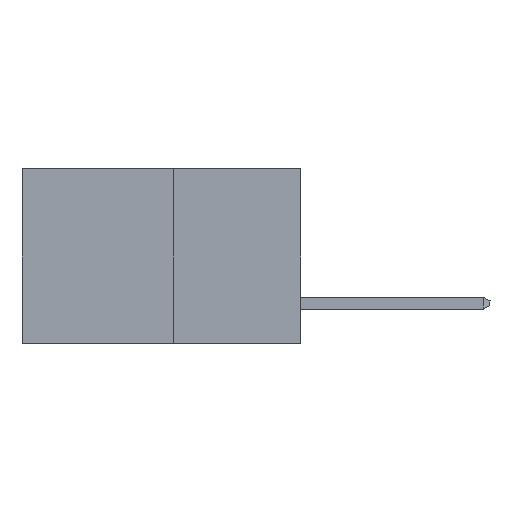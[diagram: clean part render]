
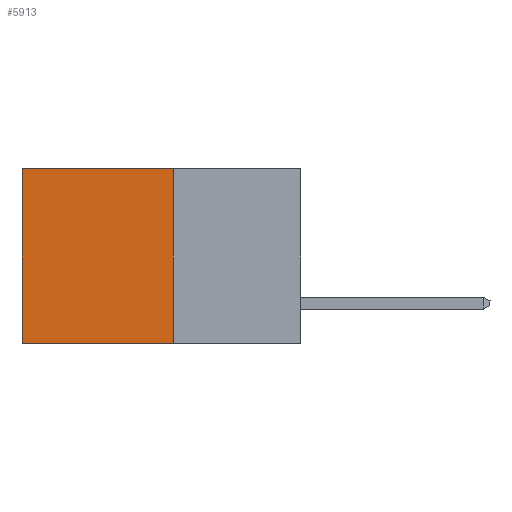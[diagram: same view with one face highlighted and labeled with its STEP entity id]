
A CAD part, left-side view. The second image highlights one B-rep face of the part: STEP entity #5913.
In plain terms, the highlighted planar face has unit normal (-1, 0, 0).
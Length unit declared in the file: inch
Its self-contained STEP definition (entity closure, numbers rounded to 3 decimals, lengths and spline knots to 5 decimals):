
#303 = CARTESIAN_POINT ( 'NONE',  ( 0.277, 0.59, 0. ) ) ;
#941 = VERTEX_POINT ( 'NONE', #5089 ) ;
#949 = LINE ( 'NONE', #4403, #7900 ) ;
#1093 = FACE_OUTER_BOUND ( 'NONE', #1578, .T. ) ;
#1366 = DIRECTION ( 'NONE',  ( 1., 0., 0. ) ) ;
#1402 = LINE ( 'NONE', #5482, #10007 ) ;
#1578 = EDGE_LOOP ( 'NONE', ( #9532, #2005, #4877, #5020 ) ) ;
#1943 = VECTOR ( 'NONE', #10013, 39.37008 ) ;
#2005 = ORIENTED_EDGE ( 'NONE', *, *, #7755, .F. ) ;
#2115 = VECTOR ( 'NONE', #4430, 39.37008 ) ;
#2219 = EDGE_CURVE ( 'NONE', #7611, #7631, #1402, .T. ) ;
#3557 = CARTESIAN_POINT ( 'NONE',  ( 0.277, 0.27, 0. ) ) ;
#3905 = CARTESIAN_POINT ( 'NONE',  ( 0.277, 0.59, -0.37 ) ) ;
#4254 = AXIS2_PLACEMENT_3D ( 'NONE', #10764, #1366, #7440 ) ;
#4403 = CARTESIAN_POINT ( 'NONE',  ( 0.277, 0.27, -0.37 ) ) ;
#4430 = DIRECTION ( 'NONE',  ( 0., 1., 0. ) ) ;
#4716 = DIRECTION ( 'NONE',  ( 0., 0., -1. ) ) ;
#4877 = ORIENTED_EDGE ( 'NONE', *, *, #6781, .F. ) ;
#5020 = ORIENTED_EDGE ( 'NONE', *, *, #5606, .T. ) ;
#5089 = CARTESIAN_POINT ( 'NONE',  ( 0.277, 0.27, -0.37 ) ) ;
#5482 = CARTESIAN_POINT ( 'NONE',  ( 0.277, 0.59, -0.37 ) ) ;
#5606 = EDGE_CURVE ( 'NONE', #9499, #7611, #6719, .T. ) ;
#5913 = ADVANCED_FACE ( 'NONE', ( #1093 ), #9934, .F. ) ;
#6719 = LINE ( 'NONE', #3557, #2115 ) ;
#6781 = EDGE_CURVE ( 'NONE', #9499, #941, #949, .T. ) ;
#7075 = LINE ( 'NONE', #10840, #1943 ) ;
#7264 = CARTESIAN_POINT ( 'NONE',  ( 0.277, 0.27, 0. ) ) ;
#7440 = DIRECTION ( 'NONE',  ( 0., 0., -1. ) ) ;
#7611 = VERTEX_POINT ( 'NONE', #303 ) ;
#7631 = VERTEX_POINT ( 'NONE', #3905 ) ;
#7755 = EDGE_CURVE ( 'NONE', #941, #7631, #7075, .T. ) ;
#7803 = DIRECTION ( 'NONE',  ( 0., 0., -1. ) ) ;
#7900 = VECTOR ( 'NONE', #7803, 39.37008 ) ;
#9499 = VERTEX_POINT ( 'NONE', #7264 ) ;
#9532 = ORIENTED_EDGE ( 'NONE', *, *, #2219, .T. ) ;
#9934 = PLANE ( 'NONE',  #4254 ) ;
#10007 = VECTOR ( 'NONE', #4716, 39.37008 ) ;
#10013 = DIRECTION ( 'NONE',  ( 0., 1., 0. ) ) ;
#10764 = CARTESIAN_POINT ( 'NONE',  ( 0.277, 0.27, -0.37 ) ) ;
#10840 = CARTESIAN_POINT ( 'NONE',  ( 0.277, 0.27, -0.37 ) ) ;
